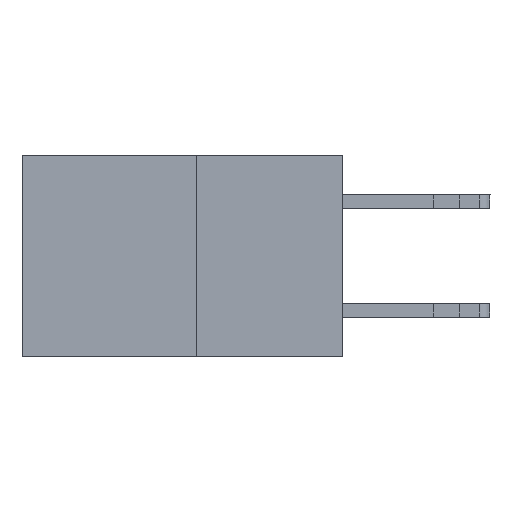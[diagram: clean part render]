
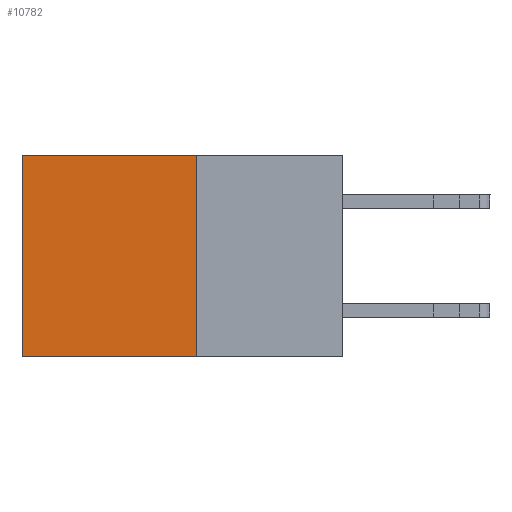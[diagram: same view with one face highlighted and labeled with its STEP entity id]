
A CAD part, left-side view. The second image highlights one B-rep face of the part: STEP entity #10782.
In plain terms, the highlighted planar face has unit normal (-1, 0, 0).
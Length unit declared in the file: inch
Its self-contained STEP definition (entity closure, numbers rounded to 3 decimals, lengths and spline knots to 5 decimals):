
#651 = VECTOR ( 'NONE', #3607, 39.37008 ) ;
#1439 = DIRECTION ( 'NONE',  ( 0., 0., -1. ) ) ;
#2042 = DIRECTION ( 'NONE',  ( 1., 0., 0. ) ) ;
#2701 = CARTESIAN_POINT ( 'NONE',  ( 0.277, 0.59, 0. ) ) ;
#2901 = CARTESIAN_POINT ( 'NONE',  ( 0.277, 0.27, 0. ) ) ;
#2940 = VECTOR ( 'NONE', #14379, 39.37008 ) ;
#3607 = DIRECTION ( 'NONE',  ( 0., 1., 0. ) ) ;
#4036 = FACE_OUTER_BOUND ( 'NONE', #16234, .T. ) ;
#4376 = VERTEX_POINT ( 'NONE', #9070 ) ;
#4982 = EDGE_CURVE ( 'NONE', #8773, #4376, #6437, .T. ) ;
#5099 = CARTESIAN_POINT ( 'NONE',  ( 0.277, 0.59, -0.37 ) ) ;
#5243 = VECTOR ( 'NONE', #1439, 39.37008 ) ;
#5492 = PLANE ( 'NONE',  #14664 ) ;
#5808 = CARTESIAN_POINT ( 'NONE',  ( 0.277, 0.27, -0.37 ) ) ;
#6437 = LINE ( 'NONE', #5099, #5243 ) ;
#7914 = ORIENTED_EDGE ( 'NONE', *, *, #21150, .F. ) ;
#8773 = VERTEX_POINT ( 'NONE', #2701 ) ;
#9070 = CARTESIAN_POINT ( 'NONE',  ( 0.277, 0.59, -0.37 ) ) ;
#9278 = CARTESIAN_POINT ( 'NONE',  ( 0.277, 0.27, -0.37 ) ) ;
#9637 = EDGE_CURVE ( 'NONE', #21329, #4376, #19211, .T. ) ;
#9681 = ORIENTED_EDGE ( 'NONE', *, *, #15019, .T. ) ;
#10572 = VERTEX_POINT ( 'NONE', #2901 ) ;
#10782 = ADVANCED_FACE ( 'NONE', ( #4036 ), #5492, .F. ) ;
#12043 = LINE ( 'NONE', #13600, #651 ) ;
#13600 = CARTESIAN_POINT ( 'NONE',  ( 0.277, 0.27, 0. ) ) ;
#13979 = DIRECTION ( 'NONE',  ( 0., 0., -1. ) ) ;
#14256 = ORIENTED_EDGE ( 'NONE', *, *, #4982, .T. ) ;
#14379 = DIRECTION ( 'NONE',  ( 0., 1., 0. ) ) ;
#14664 = AXIS2_PLACEMENT_3D ( 'NONE', #5808, #2042, #17651 ) ;
#14857 = ORIENTED_EDGE ( 'NONE', *, *, #9637, .F. ) ;
#15019 = EDGE_CURVE ( 'NONE', #10572, #8773, #12043, .T. ) ;
#15732 = CARTESIAN_POINT ( 'NONE',  ( 0.277, 0.27, -0.37 ) ) ;
#16234 = EDGE_LOOP ( 'NONE', ( #14256, #14857, #7914, #9681 ) ) ;
#17651 = DIRECTION ( 'NONE',  ( 0., 0., -1. ) ) ;
#18707 = LINE ( 'NONE', #15732, #20589 ) ;
#19211 = LINE ( 'NONE', #9278, #2940 ) ;
#20589 = VECTOR ( 'NONE', #13979, 39.37008 ) ;
#20905 = CARTESIAN_POINT ( 'NONE',  ( 0.277, 0.27, -0.37 ) ) ;
#21150 = EDGE_CURVE ( 'NONE', #10572, #21329, #18707, .T. ) ;
#21329 = VERTEX_POINT ( 'NONE', #20905 ) ;
